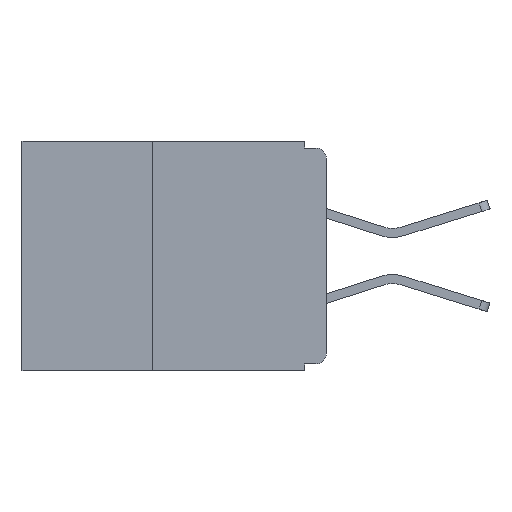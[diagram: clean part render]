
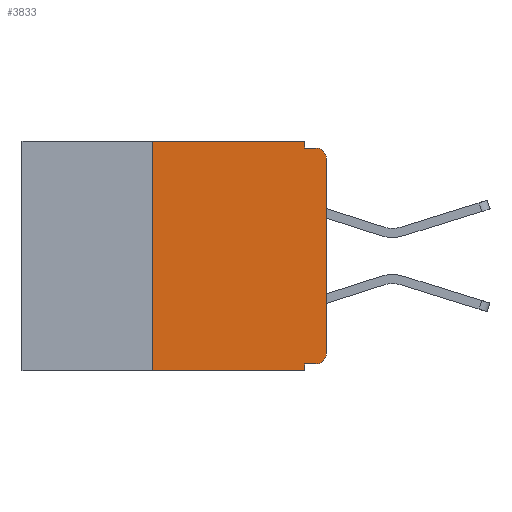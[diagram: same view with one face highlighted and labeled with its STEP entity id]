
A CAD part, left-side view. The second image highlights one B-rep face of the part: STEP entity #3833.
In plain terms, the highlighted planar face has unit normal (-1, 0, 0).
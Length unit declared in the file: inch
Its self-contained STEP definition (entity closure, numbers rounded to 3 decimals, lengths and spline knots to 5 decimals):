
#77 = ORIENTED_EDGE ( 'NONE', *, *, #35020, .T. ) ;
#92 = DIRECTION ( 'NONE',  ( 1., 0., 0. ) ) ;
#326 = CARTESIAN_POINT ( 'NONE',  ( 0., 0., -0.025 ) ) ;
#937 = ORIENTED_EDGE ( 'NONE', *, *, #3502, .T. ) ;
#1141 = CARTESIAN_POINT ( 'NONE',  ( 0., 0.031, 0. ) ) ;
#1246 = ORIENTED_EDGE ( 'NONE', *, *, #25989, .F. ) ;
#1272 = DIRECTION ( 'NONE',  ( 0., -1., 0. ) ) ;
#1283 = ORIENTED_EDGE ( 'NONE', *, *, #25734, .F. ) ;
#1689 = ORIENTED_EDGE ( 'NONE', *, *, #15122, .F. ) ;
#1735 = CARTESIAN_POINT ( 'NONE',  ( 0., 0., -0.305 ) ) ;
#1809 = ORIENTED_EDGE ( 'NONE', *, *, #23915, .F. ) ;
#1845 = ORIENTED_EDGE ( 'NONE', *, *, #20250, .T. ) ;
#2164 = ORIENTED_EDGE ( 'NONE', *, *, #18457, .F. ) ;
#2814 = ORIENTED_EDGE ( 'NONE', *, *, #7372, .F. ) ;
#3269 = VECTOR ( 'NONE', #1272, 39.37008 ) ;
#3502 = EDGE_CURVE ( 'NONE', #26212, #23481, #31745, .T. ) ;
#3509 = ORIENTED_EDGE ( 'NONE', *, *, #26651, .T. ) ;
#3833 = ADVANCED_FACE ( 'NONE', ( #6647 ), #17130, .F. ) ;
#5030 = LINE ( 'NONE', #23581, #33543 ) ;
#5084 = LINE ( 'NONE', #13076, #10017 ) ;
#5634 = CARTESIAN_POINT ( 'NONE',  ( 0., 0.015, -0.305 ) ) ;
#6623 = LINE ( 'NONE', #13403, #11138 ) ;
#6647 = FACE_OUTER_BOUND ( 'NONE', #30071, .T. ) ;
#6861 = VERTEX_POINT ( 'NONE', #1735 ) ;
#7372 = EDGE_CURVE ( 'NONE', #27881, #30533, #5030, .T. ) ;
#8542 = DIRECTION ( 'NONE',  ( 0., 0., -1. ) ) ;
#8799 = VERTEX_POINT ( 'NONE', #21150 ) ;
#9132 = VERTEX_POINT ( 'NONE', #33303 ) ;
#9719 = CARTESIAN_POINT ( 'NONE',  ( 0., 0.031, -0.33 ) ) ;
#10017 = VECTOR ( 'NONE', #29458, 39.37008 ) ;
#10580 = DIRECTION ( 'NONE',  ( 0., 0., 1. ) ) ;
#11138 = VECTOR ( 'NONE', #32490, 39.37008 ) ;
#12183 = CARTESIAN_POINT ( 'NONE',  ( 0., 0.031, -0.01 ) ) ;
#12960 = CARTESIAN_POINT ( 'NONE',  ( 0., 0.015, -0.025 ) ) ;
#13076 = CARTESIAN_POINT ( 'NONE',  ( 0., 0.031, -0.33 ) ) ;
#13403 = CARTESIAN_POINT ( 'NONE',  ( 0., 0.25, -0.33 ) ) ;
#13491 = VERTEX_POINT ( 'NONE', #9719 ) ;
#14160 = CARTESIAN_POINT ( 'NONE',  ( 0., 0.015, -0.01 ) ) ;
#15122 = EDGE_CURVE ( 'NONE', #33556, #9132, #19403, .T. ) ;
#15794 = DIRECTION ( 'NONE',  ( 0., 0., -1. ) ) ;
#16820 = CIRCLE ( 'NONE', #23859, 0.015 ) ;
#17130 = PLANE ( 'NONE',  #17645 ) ;
#17645 = AXIS2_PLACEMENT_3D ( 'NONE', #28027, #92, #19971 ) ;
#18457 = EDGE_CURVE ( 'NONE', #30533, #13491, #5084, .T. ) ;
#18872 = VERTEX_POINT ( 'NONE', #12183 ) ;
#19403 = LINE ( 'NONE', #21107, #32953 ) ;
#19971 = DIRECTION ( 'NONE',  ( 0., 0., -1. ) ) ;
#20250 = EDGE_CURVE ( 'NONE', #8799, #13491, #26431, .T. ) ;
#21107 = CARTESIAN_POINT ( 'NONE',  ( 0., 0.437, 0. ) ) ;
#21150 = CARTESIAN_POINT ( 'NONE',  ( 0., 0.25, -0.33 ) ) ;
#23481 = VERTEX_POINT ( 'NONE', #14160 ) ;
#23581 = CARTESIAN_POINT ( 'NONE',  ( 0., 0., -0.32 ) ) ;
#23850 = DIRECTION ( 'NONE',  ( 0., -1., 0. ) ) ;
#23859 = AXIS2_PLACEMENT_3D ( 'NONE', #5634, #25162, #8542 ) ;
#23915 = EDGE_CURVE ( 'NONE', #8799, #33556, #6623, .T. ) ;
#24534 = VECTOR ( 'NONE', #32752, 39.37008 ) ;
#25162 = DIRECTION ( 'NONE',  ( -1., 0., 0. ) ) ;
#25345 = CARTESIAN_POINT ( 'NONE',  ( 0., 0.015, -0.32 ) ) ;
#25368 = LINE ( 'NONE', #35456, #24534 ) ;
#25411 = VECTOR ( 'NONE', #10580, 39.37008 ) ;
#25734 = EDGE_CURVE ( 'NONE', #9132, #18872, #26644, .T. ) ;
#25805 = VECTOR ( 'NONE', #29102, 39.37008 ) ;
#25989 = EDGE_CURVE ( 'NONE', #18872, #23481, #25368, .T. ) ;
#26212 = VERTEX_POINT ( 'NONE', #326 ) ;
#26311 = DIRECTION ( 'NONE',  ( 0., 1., 0. ) ) ;
#26431 = LINE ( 'NONE', #34523, #3269 ) ;
#26644 = LINE ( 'NONE', #1141, #25805 ) ;
#26651 = EDGE_CURVE ( 'NONE', #27881, #6861, #16820, .T. ) ;
#27060 = CARTESIAN_POINT ( 'NONE',  ( 0., 0., 0. ) ) ;
#27759 = CARTESIAN_POINT ( 'NONE',  ( 0., 0.031, -0.32 ) ) ;
#27881 = VERTEX_POINT ( 'NONE', #25345 ) ;
#28012 = CARTESIAN_POINT ( 'NONE',  ( 0., 0.25, 0. ) ) ;
#28027 = CARTESIAN_POINT ( 'NONE',  ( 0., 0.437, 0. ) ) ;
#29102 = DIRECTION ( 'NONE',  ( 0., 0., -1. ) ) ;
#29458 = DIRECTION ( 'NONE',  ( 0., 0., -1. ) ) ;
#30071 = EDGE_LOOP ( 'NONE', ( #77, #937, #1246, #1283, #1689, #1809, #1845, #2164, #2814, #3509 ) ) ;
#30533 = VERTEX_POINT ( 'NONE', #27759 ) ;
#31745 = CIRCLE ( 'NONE', #34826, 0.015 ) ;
#32066 = DIRECTION ( 'NONE',  ( -1., 0., 0. ) ) ;
#32490 = DIRECTION ( 'NONE',  ( 0., 0., 1. ) ) ;
#32582 = LINE ( 'NONE', #27060, #25411 ) ;
#32752 = DIRECTION ( 'NONE',  ( 0., -1., 0. ) ) ;
#32953 = VECTOR ( 'NONE', #23850, 39.37008 ) ;
#33303 = CARTESIAN_POINT ( 'NONE',  ( 0., 0.031, 0. ) ) ;
#33543 = VECTOR ( 'NONE', #26311, 39.37008 ) ;
#33556 = VERTEX_POINT ( 'NONE', #28012 ) ;
#34523 = CARTESIAN_POINT ( 'NONE',  ( 0., 0.437, -0.33 ) ) ;
#34826 = AXIS2_PLACEMENT_3D ( 'NONE', #12960, #32066, #15794 ) ;
#35020 = EDGE_CURVE ( 'NONE', #6861, #26212, #32582, .T. ) ;
#35456 = CARTESIAN_POINT ( 'NONE',  ( 0., 0., -0.01 ) ) ;
